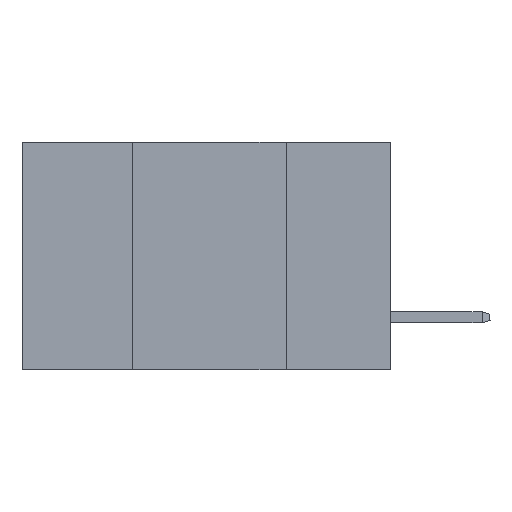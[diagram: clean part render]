
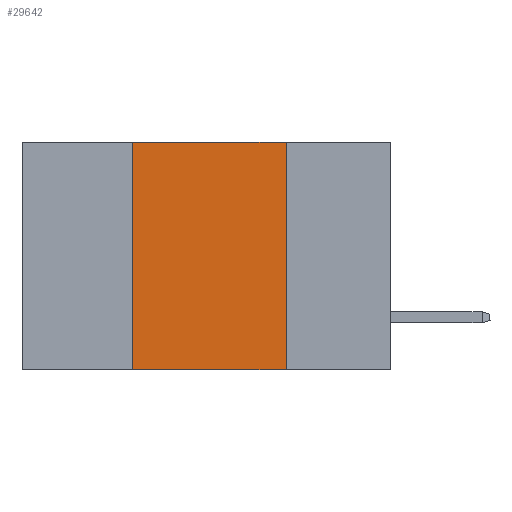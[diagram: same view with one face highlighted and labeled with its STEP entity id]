
A CAD part, left-side view. The second image highlights one B-rep face of the part: STEP entity #29642.
In plain terms, the highlighted planar face has unit normal (-1, 0, 0).
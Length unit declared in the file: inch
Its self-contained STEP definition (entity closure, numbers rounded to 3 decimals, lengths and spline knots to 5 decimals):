
#1662 = VECTOR ( 'NONE', #7240, 39.37008 ) ;
#2035 = EDGE_CURVE ( 'NONE', #25939, #5731, #17319, .T. ) ;
#2291 = PLANE ( 'NONE',  #6971 ) ;
#2937 = CARTESIAN_POINT ( 'NONE',  ( 0., 0.42, 0. ) ) ;
#5117 = VERTEX_POINT ( 'NONE', #22148 ) ;
#5731 = VERTEX_POINT ( 'NONE', #27344 ) ;
#6971 = AXIS2_PLACEMENT_3D ( 'NONE', #10477, #7485, #31151 ) ;
#7240 = DIRECTION ( 'NONE',  ( 0., -1., 0. ) ) ;
#7276 = CARTESIAN_POINT ( 'NONE',  ( 0., 0.17, 0. ) ) ;
#7485 = DIRECTION ( 'NONE',  ( 1., 0., 0. ) ) ;
#7740 = DIRECTION ( 'NONE',  ( 0., 0., -1. ) ) ;
#8078 = VECTOR ( 'NONE', #29040, 39.37008 ) ;
#9599 = CARTESIAN_POINT ( 'NONE',  ( 0., 0.42, -0.37 ) ) ;
#9679 = EDGE_CURVE ( 'NONE', #19067, #5117, #33748, .T. ) ;
#9942 = ORIENTED_EDGE ( 'NONE', *, *, #18824, .F. ) ;
#10477 = CARTESIAN_POINT ( 'NONE',  ( 0., 0.6, 0. ) ) ;
#10920 = LINE ( 'NONE', #7276, #21265 ) ;
#14935 = ORIENTED_EDGE ( 'NONE', *, *, #19448, .F. ) ;
#16464 = DIRECTION ( 'NONE',  ( 0., -1., 0. ) ) ;
#17319 = LINE ( 'NONE', #17734, #1662 ) ;
#17734 = CARTESIAN_POINT ( 'NONE',  ( 0., 0.6, -0.37 ) ) ;
#18824 = EDGE_CURVE ( 'NONE', #25939, #19067, #26685, .T. ) ;
#19067 = VERTEX_POINT ( 'NONE', #25072 ) ;
#19448 = EDGE_CURVE ( 'NONE', #5117, #5731, #10920, .T. ) ;
#20082 = VECTOR ( 'NONE', #16464, 39.37008 ) ;
#21093 = EDGE_LOOP ( 'NONE', ( #14935, #25329, #9942, #31338 ) ) ;
#21265 = VECTOR ( 'NONE', #7740, 39.37008 ) ;
#22065 = FACE_OUTER_BOUND ( 'NONE', #21093, .T. ) ;
#22148 = CARTESIAN_POINT ( 'NONE',  ( 0., 0.17, 0. ) ) ;
#25072 = CARTESIAN_POINT ( 'NONE',  ( 0., 0.42, 0. ) ) ;
#25329 = ORIENTED_EDGE ( 'NONE', *, *, #9679, .F. ) ;
#25939 = VERTEX_POINT ( 'NONE', #9599 ) ;
#26685 = LINE ( 'NONE', #2937, #8078 ) ;
#27344 = CARTESIAN_POINT ( 'NONE',  ( 0., 0.17, -0.37 ) ) ;
#27357 = CARTESIAN_POINT ( 'NONE',  ( 0., 0.6, 0. ) ) ;
#29040 = DIRECTION ( 'NONE',  ( 0., 0., 1. ) ) ;
#29642 = ADVANCED_FACE ( 'NONE', ( #22065 ), #2291, .F. ) ;
#31151 = DIRECTION ( 'NONE',  ( 0., 0., -1. ) ) ;
#31338 = ORIENTED_EDGE ( 'NONE', *, *, #2035, .T. ) ;
#33748 = LINE ( 'NONE', #27357, #20082 ) ;
